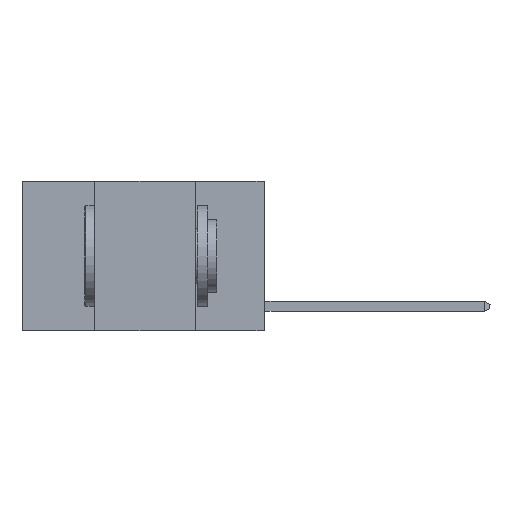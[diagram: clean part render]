
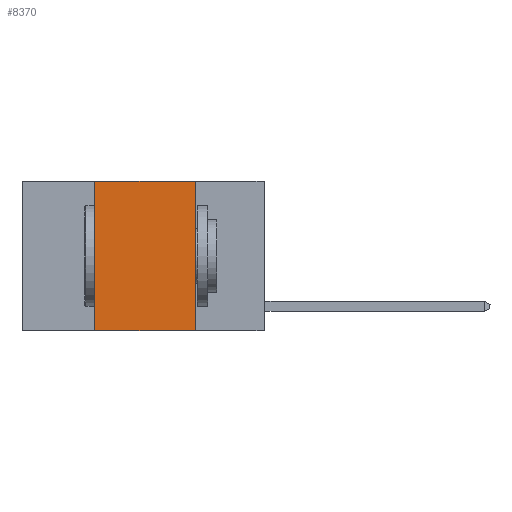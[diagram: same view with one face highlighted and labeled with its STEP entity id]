
A CAD part, left-side view. The second image highlights one B-rep face of the part: STEP entity #8370.
In plain terms, the highlighted planar face has unit normal (-1, 0, 0).
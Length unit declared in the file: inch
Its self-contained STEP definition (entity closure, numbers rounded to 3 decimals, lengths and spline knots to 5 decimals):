
#55 = VERTEX_POINT ( 'NONE', #19611 ) ;
#272 = VECTOR ( 'NONE', #17836, 39.37008 ) ;
#944 = DIRECTION ( 'NONE',  ( 0., 0., -1. ) ) ;
#1489 = EDGE_CURVE ( 'NONE', #20244, #55, #27159, .T. ) ;
#3661 = PLANE ( 'NONE',  #8690 ) ;
#4664 = EDGE_CURVE ( 'NONE', #11094, #55, #16934, .T. ) ;
#4893 = CARTESIAN_POINT ( 'NONE',  ( 0., 0.6, -0.37 ) ) ;
#6095 = CARTESIAN_POINT ( 'NONE',  ( 0., 0.17, 0. ) ) ;
#6717 = VECTOR ( 'NONE', #15281, 39.37008 ) ;
#6950 = VECTOR ( 'NONE', #19027, 39.37008 ) ;
#8370 = ADVANCED_FACE ( 'NONE', ( #12565 ), #3661, .F. ) ;
#8629 = VERTEX_POINT ( 'NONE', #11944 ) ;
#8645 = ORIENTED_EDGE ( 'NONE', *, *, #22342, .F. ) ;
#8690 = AXIS2_PLACEMENT_3D ( 'NONE', #10601, #29089, #944 ) ;
#10601 = CARTESIAN_POINT ( 'NONE',  ( 0., 0.6, 0. ) ) ;
#10788 = LINE ( 'NONE', #22799, #272 ) ;
#11094 = VERTEX_POINT ( 'NONE', #21691 ) ;
#11944 = CARTESIAN_POINT ( 'NONE',  ( 0., 0.42, 0. ) ) ;
#12565 = FACE_OUTER_BOUND ( 'NONE', #29530, .T. ) ;
#15132 = EDGE_CURVE ( 'NONE', #8629, #20244, #10788, .T. ) ;
#15191 = ORIENTED_EDGE ( 'NONE', *, *, #4664, .T. ) ;
#15281 = DIRECTION ( 'NONE',  ( 0., 0., -1. ) ) ;
#16696 = LINE ( 'NONE', #25856, #28477 ) ;
#16934 = LINE ( 'NONE', #4893, #6950 ) ;
#17396 = ORIENTED_EDGE ( 'NONE', *, *, #1489, .F. ) ;
#17836 = DIRECTION ( 'NONE',  ( 0., -1., 0. ) ) ;
#19027 = DIRECTION ( 'NONE',  ( 0., -1., 0. ) ) ;
#19611 = CARTESIAN_POINT ( 'NONE',  ( 0., 0.17, -0.37 ) ) ;
#20244 = VERTEX_POINT ( 'NONE', #25622 ) ;
#21691 = CARTESIAN_POINT ( 'NONE',  ( 0., 0.42, -0.37 ) ) ;
#22342 = EDGE_CURVE ( 'NONE', #11094, #8629, #16696, .T. ) ;
#22799 = CARTESIAN_POINT ( 'NONE',  ( 0., 0.6, 0. ) ) ;
#23591 = DIRECTION ( 'NONE',  ( 0., 0., 1. ) ) ;
#24555 = ORIENTED_EDGE ( 'NONE', *, *, #15132, .F. ) ;
#25622 = CARTESIAN_POINT ( 'NONE',  ( 0., 0.17, 0. ) ) ;
#25856 = CARTESIAN_POINT ( 'NONE',  ( 0., 0.42, 0. ) ) ;
#27159 = LINE ( 'NONE', #6095, #6717 ) ;
#28477 = VECTOR ( 'NONE', #23591, 39.37008 ) ;
#29089 = DIRECTION ( 'NONE',  ( 1., 0., 0. ) ) ;
#29530 = EDGE_LOOP ( 'NONE', ( #17396, #24555, #8645, #15191 ) ) ;
